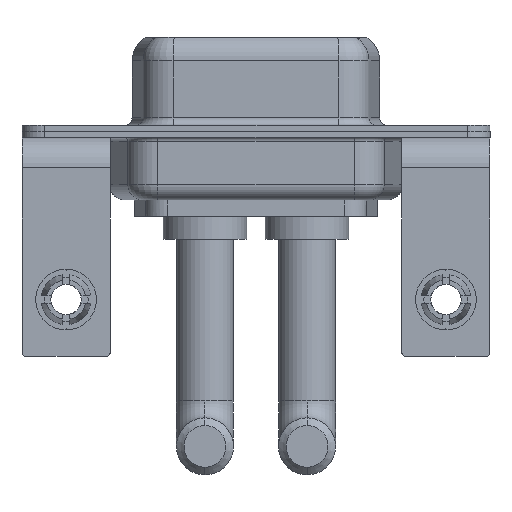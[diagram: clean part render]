
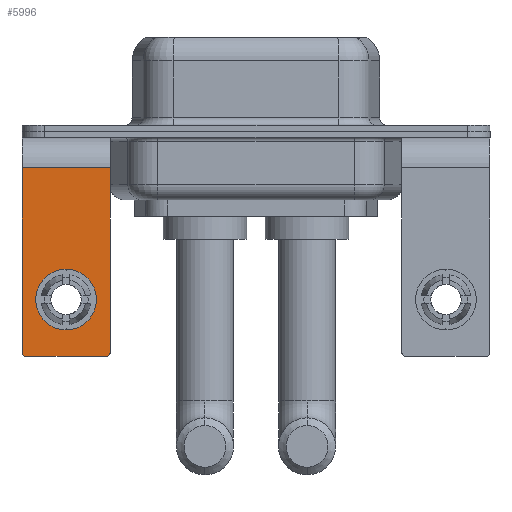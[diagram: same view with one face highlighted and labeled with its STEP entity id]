
A CAD part, front view. The second image highlights one B-rep face of the part: STEP entity #5996.
In plain terms, the highlighted planar face has unit normal (0, -1, 0).
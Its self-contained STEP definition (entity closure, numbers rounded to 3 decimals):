
#97 = ORIENTED_EDGE ( 'NONE', *, *, #13065, .T. ) ;
#271 = CARTESIAN_POINT ( 'NONE',  ( 0., -6.25, -11.07 ) ) ;
#393 = DIRECTION ( 'NONE',  ( 0., 0., 1. ) ) ;
#1050 = PLANE ( 'NONE',  #1740 ) ;
#1180 = FACE_OUTER_BOUND ( 'NONE', #6515, .T. ) ;
#1370 = EDGE_CURVE ( 'NONE', #3906, #8455, #7557, .T. ) ;
#1401 = VECTOR ( 'NONE', #9302, 1000. ) ;
#1740 = AXIS2_PLACEMENT_3D ( 'NONE', #4449, #11423, #4586 ) ;
#1776 = DIRECTION ( 'NONE',  ( 0., -1., 0. ) ) ;
#1795 = CARTESIAN_POINT ( 'NONE',  ( 2.9, -6.25, -2.4 ) ) ;
#1989 = CARTESIAN_POINT ( 'NONE',  ( 2.9, -6.25, -14.8 ) ) ;
#2242 = VERTEX_POINT ( 'NONE', #7740 ) ;
#2452 = CIRCLE ( 'NONE', #2931, 0.25 ) ;
#2618 = CARTESIAN_POINT ( 'NONE',  ( 2.9, -6.25, -2.4 ) ) ;
#2860 = AXIS2_PLACEMENT_3D ( 'NONE', #271, #9045, #4624 ) ;
#2931 = AXIS2_PLACEMENT_3D ( 'NONE', #11877, #1776, #6285 ) ;
#3035 = EDGE_CURVE ( 'NONE', #11119, #2242, #6245, .T. ) ;
#3116 = ORIENTED_EDGE ( 'NONE', *, *, #3035, .T. ) ;
#3301 = CARTESIAN_POINT ( 'NONE',  ( 2.9, -6.25, -14.55 ) ) ;
#3313 = VECTOR ( 'NONE', #14144, 1000. ) ;
#3472 = VERTEX_POINT ( 'NONE', #8457 ) ;
#3511 = DIRECTION ( 'NONE',  ( 0., -1., 0. ) ) ;
#3906 = VERTEX_POINT ( 'NONE', #13647 ) ;
#4449 = CARTESIAN_POINT ( 'NONE',  ( 2.9, -6.25, -2.4 ) ) ;
#4532 = ORIENTED_EDGE ( 'NONE', *, *, #9863, .T. ) ;
#4586 = DIRECTION ( 'NONE',  ( 0., 0., 1. ) ) ;
#4587 = CARTESIAN_POINT ( 'NONE',  ( 2.9, -6.25, -2.4 ) ) ;
#4595 = EDGE_CURVE ( 'NONE', #2242, #3472, #2452, .T. ) ;
#4624 = DIRECTION ( 'NONE',  ( 0., 0., 1. ) ) ;
#5140 = VERTEX_POINT ( 'NONE', #1795 ) ;
#5952 = CARTESIAN_POINT ( 'NONE',  ( -2.9, -6.25, -2.4 ) ) ;
#5995 = CARTESIAN_POINT ( 'NONE',  ( 0., -6.25, -11.07 ) ) ;
#5996 = ADVANCED_FACE ( 'NONE', ( #12528, #1180 ), #1050, .F. ) ;
#6016 = LINE ( 'NONE', #2618, #13862 ) ;
#6245 = LINE ( 'NONE', #5952, #7615 ) ;
#6285 = DIRECTION ( 'NONE',  ( 0., 0., 1. ) ) ;
#6432 = ORIENTED_EDGE ( 'NONE', *, *, #10766, .F. ) ;
#6515 = EDGE_LOOP ( 'NONE', ( #3116, #11343, #6432, #97, #14211, #10534 ) ) ;
#6816 = CIRCLE ( 'NONE', #10117, 0.25 ) ;
#7240 = DIRECTION ( 'NONE',  ( 0., 1., 0. ) ) ;
#7557 = CIRCLE ( 'NONE', #2860, 2. ) ;
#7615 = VECTOR ( 'NONE', #10591, 1000. ) ;
#7740 = CARTESIAN_POINT ( 'NONE',  ( -2.9, -6.25, -14.55 ) ) ;
#7902 = VERTEX_POINT ( 'NONE', #3301 ) ;
#8035 = LINE ( 'NONE', #4587, #1401 ) ;
#8247 = ORIENTED_EDGE ( 'NONE', *, *, #1370, .T. ) ;
#8455 = VERTEX_POINT ( 'NONE', #11935 ) ;
#8457 = CARTESIAN_POINT ( 'NONE',  ( -2.65, -6.25, -14.8 ) ) ;
#8654 = VERTEX_POINT ( 'NONE', #11129 ) ;
#9045 = DIRECTION ( 'NONE',  ( 0., 1., 0. ) ) ;
#9140 = CIRCLE ( 'NONE', #10084, 2. ) ;
#9302 = DIRECTION ( 'NONE',  ( 0., 0., -1. ) ) ;
#9475 = EDGE_LOOP ( 'NONE', ( #4532, #8247 ) ) ;
#9863 = EDGE_CURVE ( 'NONE', #8455, #3906, #9140, .T. ) ;
#10084 = AXIS2_PLACEMENT_3D ( 'NONE', #5995, #7240, #393 ) ;
#10117 = AXIS2_PLACEMENT_3D ( 'NONE', #14479, #3511, #12494 ) ;
#10462 = CARTESIAN_POINT ( 'NONE',  ( -2.9, -6.25, -2.4 ) ) ;
#10508 = DIRECTION ( 'NONE',  ( -1., 0., 0. ) ) ;
#10534 = ORIENTED_EDGE ( 'NONE', *, *, #13180, .T. ) ;
#10591 = DIRECTION ( 'NONE',  ( 0., 0., -1. ) ) ;
#10766 = EDGE_CURVE ( 'NONE', #8654, #3472, #12170, .T. ) ;
#11119 = VERTEX_POINT ( 'NONE', #10462 ) ;
#11129 = CARTESIAN_POINT ( 'NONE',  ( 2.65, -6.25, -14.8 ) ) ;
#11343 = ORIENTED_EDGE ( 'NONE', *, *, #4595, .T. ) ;
#11423 = DIRECTION ( 'NONE',  ( 0., 1., 0. ) ) ;
#11877 = CARTESIAN_POINT ( 'NONE',  ( -2.65, -6.25, -14.55 ) ) ;
#11935 = CARTESIAN_POINT ( 'NONE',  ( 0., -6.25, -13.07 ) ) ;
#12170 = LINE ( 'NONE', #1989, #3313 ) ;
#12494 = DIRECTION ( 'NONE',  ( 0., 0., 1. ) ) ;
#12528 = FACE_BOUND ( 'NONE', #9475, .T. ) ;
#13065 = EDGE_CURVE ( 'NONE', #8654, #7902, #6816, .T. ) ;
#13180 = EDGE_CURVE ( 'NONE', #5140, #11119, #6016, .T. ) ;
#13459 = EDGE_CURVE ( 'NONE', #5140, #7902, #8035, .T. ) ;
#13647 = CARTESIAN_POINT ( 'NONE',  ( 0., -6.25, -9.07 ) ) ;
#13862 = VECTOR ( 'NONE', #10508, 1000. ) ;
#14144 = DIRECTION ( 'NONE',  ( -1., 0., 0. ) ) ;
#14211 = ORIENTED_EDGE ( 'NONE', *, *, #13459, .F. ) ;
#14479 = CARTESIAN_POINT ( 'NONE',  ( 2.65, -6.25, -14.55 ) ) ;
